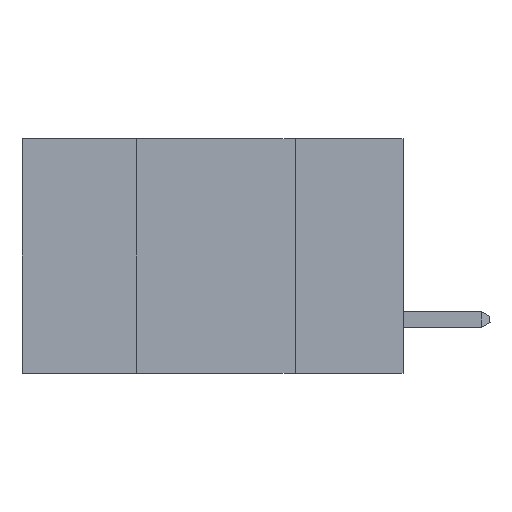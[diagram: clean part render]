
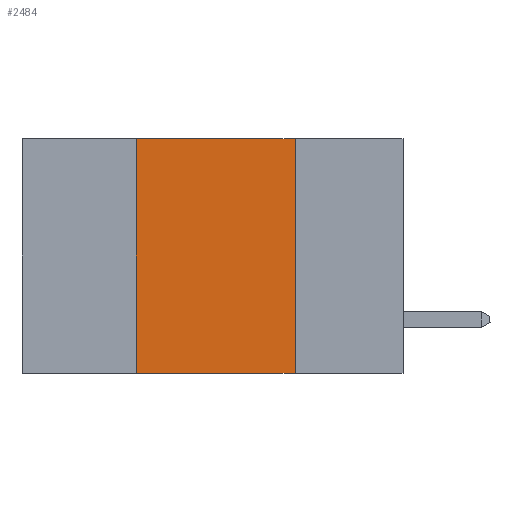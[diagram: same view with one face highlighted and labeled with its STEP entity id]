
A CAD part, left-side view. The second image highlights one B-rep face of the part: STEP entity #2484.
In plain terms, the highlighted planar face has unit normal (-1, 0, 0).
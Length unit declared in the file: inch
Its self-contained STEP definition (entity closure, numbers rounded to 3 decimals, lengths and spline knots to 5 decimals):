
#780 = VERTEX_POINT ( 'NONE', #5370 ) ;
#871 = VERTEX_POINT ( 'NONE', #3956 ) ;
#1145 = VECTOR ( 'NONE', #6741, 39.37008 ) ;
#1592 = AXIS2_PLACEMENT_3D ( 'NONE', #2680, #9302, #4374 ) ;
#2484 = ADVANCED_FACE ( 'NONE', ( #5445 ), #5188, .F. ) ;
#2680 = CARTESIAN_POINT ( 'NONE',  ( 0., 0.6, 0. ) ) ;
#3342 = LINE ( 'NONE', #9761, #5429 ) ;
#3364 = LINE ( 'NONE', #10130, #1145 ) ;
#3453 = ORIENTED_EDGE ( 'NONE', *, *, #7397, .F. ) ;
#3956 = CARTESIAN_POINT ( 'NONE',  ( 0., 0.17, 0. ) ) ;
#3972 = DIRECTION ( 'NONE',  ( 0., 0., 1. ) ) ;
#4029 = ORIENTED_EDGE ( 'NONE', *, *, #6584, .F. ) ;
#4369 = VERTEX_POINT ( 'NONE', #10657 ) ;
#4374 = DIRECTION ( 'NONE',  ( 0., 0., -1. ) ) ;
#5188 = PLANE ( 'NONE',  #1592 ) ;
#5218 = EDGE_LOOP ( 'NONE', ( #4029, #3453, #7738, #10501 ) ) ;
#5370 = CARTESIAN_POINT ( 'NONE',  ( 0., 0.17, -0.37 ) ) ;
#5429 = VECTOR ( 'NONE', #3972, 39.37008 ) ;
#5445 = FACE_OUTER_BOUND ( 'NONE', #5218, .T. ) ;
#5606 = CARTESIAN_POINT ( 'NONE',  ( 0., 0.6, -0.37 ) ) ;
#6429 = DIRECTION ( 'NONE',  ( 0., -1., 0. ) ) ;
#6439 = LINE ( 'NONE', #5606, #10438 ) ;
#6584 = EDGE_CURVE ( 'NONE', #871, #780, #3364, .T. ) ;
#6728 = CARTESIAN_POINT ( 'NONE',  ( 0., 0.42, -0.37 ) ) ;
#6741 = DIRECTION ( 'NONE',  ( 0., 0., -1. ) ) ;
#7397 = EDGE_CURVE ( 'NONE', #4369, #871, #9674, .T. ) ;
#7513 = EDGE_CURVE ( 'NONE', #8994, #4369, #3342, .T. ) ;
#7738 = ORIENTED_EDGE ( 'NONE', *, *, #7513, .F. ) ;
#7992 = DIRECTION ( 'NONE',  ( 0., -1., 0. ) ) ;
#8066 = EDGE_CURVE ( 'NONE', #8994, #780, #6439, .T. ) ;
#8502 = VECTOR ( 'NONE', #7992, 39.37008 ) ;
#8994 = VERTEX_POINT ( 'NONE', #6728 ) ;
#9302 = DIRECTION ( 'NONE',  ( 1., 0., 0. ) ) ;
#9623 = CARTESIAN_POINT ( 'NONE',  ( 0., 0.6, 0. ) ) ;
#9674 = LINE ( 'NONE', #9623, #8502 ) ;
#9761 = CARTESIAN_POINT ( 'NONE',  ( 0., 0.42, 0. ) ) ;
#10130 = CARTESIAN_POINT ( 'NONE',  ( 0., 0.17, 0. ) ) ;
#10438 = VECTOR ( 'NONE', #6429, 39.37008 ) ;
#10501 = ORIENTED_EDGE ( 'NONE', *, *, #8066, .T. ) ;
#10657 = CARTESIAN_POINT ( 'NONE',  ( 0., 0.42, 0. ) ) ;
